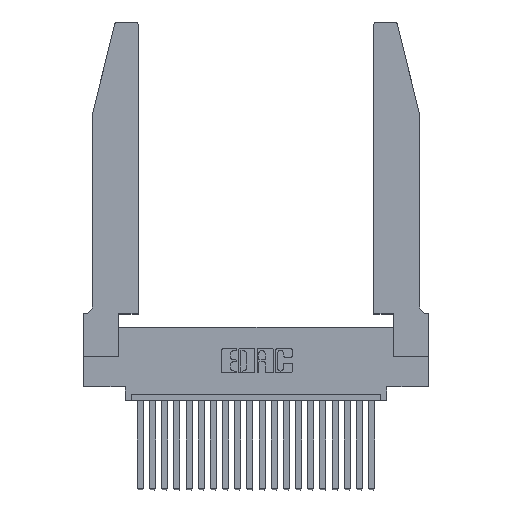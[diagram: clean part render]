
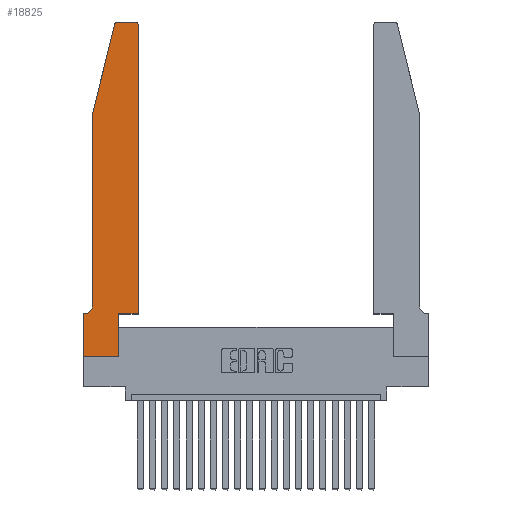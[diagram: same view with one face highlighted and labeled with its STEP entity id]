
A CAD part, top view. The second image highlights one B-rep face of the part: STEP entity #18825.
In plain terms, the highlighted planar face has unit normal (0, 0, 1).
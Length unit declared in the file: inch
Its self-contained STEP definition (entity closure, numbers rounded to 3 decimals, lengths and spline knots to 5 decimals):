
#88 = CARTESIAN_POINT ( 'NONE',  ( 0.0755, 0.35, 0.37 ) ) ;
#202 = DIRECTION ( 'NONE',  ( 0., 0., 1. ) ) ;
#567 = VERTEX_POINT ( 'NONE', #22368 ) ;
#721 = EDGE_CURVE ( 'NONE', #4636, #5144, #8232, .T. ) ;
#835 = ORIENTED_EDGE ( 'NONE', *, *, #13562, .T. ) ;
#1589 = ORIENTED_EDGE ( 'NONE', *, *, #15810, .T. ) ;
#1881 = DIRECTION ( 'NONE',  ( -1., 0., 0. ) ) ;
#1989 = DIRECTION ( 'NONE',  ( 1., 0., 0. ) ) ;
#2442 = EDGE_CURVE ( 'NONE', #5057, #567, #15553, .T. ) ;
#2459 = VERTEX_POINT ( 'NONE', #9912 ) ;
#2748 = LINE ( 'NONE', #11097, #16712 ) ;
#2771 = CARTESIAN_POINT ( 'NONE',  ( 0., 0.35, 0.37 ) ) ;
#2910 = LINE ( 'NONE', #13254, #17708 ) ;
#2966 = DIRECTION ( 'NONE',  ( 1., 0., 0. ) ) ;
#3282 = ORIENTED_EDGE ( 'NONE', *, *, #721, .T. ) ;
#3398 = ORIENTED_EDGE ( 'NONE', *, *, #12041, .T. ) ;
#3778 = DIRECTION ( 'NONE',  ( 0., 1., 0. ) ) ;
#3842 = ORIENTED_EDGE ( 'NONE', *, *, #4969, .T. ) ;
#3874 = DIRECTION ( 'NONE',  ( 0., -1., 0. ) ) ;
#4636 = VERTEX_POINT ( 'NONE', #16632 ) ;
#4881 = ORIENTED_EDGE ( 'NONE', *, *, #15313, .T. ) ;
#4969 = EDGE_CURVE ( 'NONE', #19621, #5057, #16474, .T. ) ;
#5057 = VERTEX_POINT ( 'NONE', #6912 ) ;
#5144 = VERTEX_POINT ( 'NONE', #22680 ) ;
#5571 = AXIS2_PLACEMENT_3D ( 'NONE', #6492, #18671, #2966 ) ;
#5579 = CARTESIAN_POINT ( 'NONE',  ( 0., 0., 0.37 ) ) ;
#5593 = DIRECTION ( 'NONE',  ( 1., 0., 0. ) ) ;
#5602 = AXIS2_PLACEMENT_3D ( 'NONE', #17455, #19243, #8724 ) ;
#5637 = ORIENTED_EDGE ( 'NONE', *, *, #11945, .T. ) ;
#5667 = LINE ( 'NONE', #15645, #18555 ) ;
#5780 = CARTESIAN_POINT ( 'NONE',  ( 0.4505, 0.35, 0.37 ) ) ;
#6162 = VERTEX_POINT ( 'NONE', #18208 ) ;
#6492 = CARTESIAN_POINT ( 'NONE',  ( 0.4205, 2.72, 0.37 ) ) ;
#6912 = CARTESIAN_POINT ( 'NONE',  ( 0., 0.35, 0.37 ) ) ;
#7160 = DIRECTION ( 'NONE',  ( 0., -1., 0. ) ) ;
#7289 = EDGE_LOOP ( 'NONE', ( #3398, #3282, #21137, #16554, #5637, #3842, #16510, #835, #4881, #1589, #8066, #17162 ) ) ;
#8066 = ORIENTED_EDGE ( 'NONE', *, *, #17478, .T. ) ;
#8087 = EDGE_CURVE ( 'NONE', #5144, #12531, #5667, .T. ) ;
#8232 = CIRCLE ( 'NONE', #15574, 0.03 ) ;
#8309 = VERTEX_POINT ( 'NONE', #14708 ) ;
#8505 = VECTOR ( 'NONE', #18958, 39.37008 ) ;
#8724 = DIRECTION ( 'NONE',  ( -1., 0., 0. ) ) ;
#9787 = FACE_OUTER_BOUND ( 'NONE', #7289, .T. ) ;
#9912 = CARTESIAN_POINT ( 'NONE',  ( 0.2865, 0.35, 0.37 ) ) ;
#10204 = VERTEX_POINT ( 'NONE', #16629 ) ;
#10214 = CARTESIAN_POINT ( 'NONE',  ( 0.0055, 0.35, 0.37 ) ) ;
#10587 = CIRCLE ( 'NONE', #5602, 0.07 ) ;
#10635 = LINE ( 'NONE', #11584, #18056 ) ;
#11097 = CARTESIAN_POINT ( 'NONE',  ( 0.4505, 0.35, 0.37 ) ) ;
#11243 = DIRECTION ( 'NONE',  ( 1., 0., 0. ) ) ;
#11245 = AXIS2_PLACEMENT_3D ( 'NONE', #2771, #21781, #16395 ) ;
#11485 = DIRECTION ( 'NONE',  ( -1., 0., 0. ) ) ;
#11584 = CARTESIAN_POINT ( 'NONE',  ( 0.0755, 2., 0.37 ) ) ;
#11945 = EDGE_CURVE ( 'NONE', #8309, #19621, #10587, .T. ) ;
#12041 = EDGE_CURVE ( 'NONE', #20257, #4636, #2910, .T. ) ;
#12242 = DIRECTION ( 'NONE',  ( -0.239, -0.971, 0. ) ) ;
#12531 = VERTEX_POINT ( 'NONE', #20452 ) ;
#12583 = LINE ( 'NONE', #12624, #16978 ) ;
#12624 = CARTESIAN_POINT ( 'NONE',  ( 0.4505, 0.35, 0.37 ) ) ;
#13254 = CARTESIAN_POINT ( 'NONE',  ( 0.2605, 2.75, 0.37 ) ) ;
#13562 = EDGE_CURVE ( 'NONE', #567, #10204, #22066, .T. ) ;
#14090 = CIRCLE ( 'NONE', #5571, 0.03 ) ;
#14348 = CARTESIAN_POINT ( 'NONE',  ( 0., 0., 0.37 ) ) ;
#14587 = VERTEX_POINT ( 'NONE', #5780 ) ;
#14708 = CARTESIAN_POINT ( 'NONE',  ( 0.0755, 0.42, 0.37 ) ) ;
#15161 = VECTOR ( 'NONE', #1989, 39.37008 ) ;
#15313 = EDGE_CURVE ( 'NONE', #10204, #2459, #22516, .T. ) ;
#15471 = CARTESIAN_POINT ( 'NONE',  ( 0.4205, 2.75, 0.37 ) ) ;
#15553 = LINE ( 'NONE', #14348, #18037 ) ;
#15574 = AXIS2_PLACEMENT_3D ( 'NONE', #15769, #202, #5593 ) ;
#15645 = CARTESIAN_POINT ( 'NONE',  ( 0.0755, 2., 0.37 ) ) ;
#15769 = CARTESIAN_POINT ( 'NONE',  ( 0.284, 2.72, 0.37 ) ) ;
#15810 = EDGE_CURVE ( 'NONE', #2459, #14587, #2748, .T. ) ;
#15907 = VECTOR ( 'NONE', #1881, 39.37008 ) ;
#16395 = DIRECTION ( 'NONE',  ( 1., 0., 0. ) ) ;
#16474 = LINE ( 'NONE', #88, #15907 ) ;
#16510 = ORIENTED_EDGE ( 'NONE', *, *, #2442, .T. ) ;
#16554 = ORIENTED_EDGE ( 'NONE', *, *, #18538, .T. ) ;
#16629 = CARTESIAN_POINT ( 'NONE',  ( 0.2865, 0., 0.37 ) ) ;
#16632 = CARTESIAN_POINT ( 'NONE',  ( 0.284, 2.75, 0.37 ) ) ;
#16712 = VECTOR ( 'NONE', #11243, 39.37008 ) ;
#16978 = VECTOR ( 'NONE', #3778, 39.37008 ) ;
#17162 = ORIENTED_EDGE ( 'NONE', *, *, #21169, .T. ) ;
#17455 = CARTESIAN_POINT ( 'NONE',  ( 0.0055, 0.42, 0.37 ) ) ;
#17478 = EDGE_CURVE ( 'NONE', #14587, #6162, #12583, .T. ) ;
#17708 = VECTOR ( 'NONE', #11485, 39.37008 ) ;
#18037 = VECTOR ( 'NONE', #3874, 39.37008 ) ;
#18056 = VECTOR ( 'NONE', #7160, 39.37008 ) ;
#18208 = CARTESIAN_POINT ( 'NONE',  ( 0.4505, 2.72, 0.37 ) ) ;
#18538 = EDGE_CURVE ( 'NONE', #12531, #8309, #10635, .T. ) ;
#18555 = VECTOR ( 'NONE', #12242, 39.37008 ) ;
#18671 = DIRECTION ( 'NONE',  ( 0., 0., 1. ) ) ;
#18825 = ADVANCED_FACE ( 'NONE', ( #9787 ), #22017, .T. ) ;
#18958 = DIRECTION ( 'NONE',  ( 0., 1., 0. ) ) ;
#19109 = CARTESIAN_POINT ( 'NONE',  ( 0.2865, 0.35, 0.37 ) ) ;
#19243 = DIRECTION ( 'NONE',  ( 0., 0., -1. ) ) ;
#19621 = VERTEX_POINT ( 'NONE', #10214 ) ;
#20257 = VERTEX_POINT ( 'NONE', #15471 ) ;
#20452 = CARTESIAN_POINT ( 'NONE',  ( 0.0755, 2., 0.37 ) ) ;
#21137 = ORIENTED_EDGE ( 'NONE', *, *, #8087, .T. ) ;
#21169 = EDGE_CURVE ( 'NONE', #6162, #20257, #14090, .T. ) ;
#21781 = DIRECTION ( 'NONE',  ( 0., 0., 1. ) ) ;
#22017 = PLANE ( 'NONE',  #11245 ) ;
#22066 = LINE ( 'NONE', #5579, #15161 ) ;
#22368 = CARTESIAN_POINT ( 'NONE',  ( 0., 0., 0.37 ) ) ;
#22516 = LINE ( 'NONE', #19109, #8505 ) ;
#22680 = CARTESIAN_POINT ( 'NONE',  ( 0.25487, 2.72718, 0.37 ) ) ;
